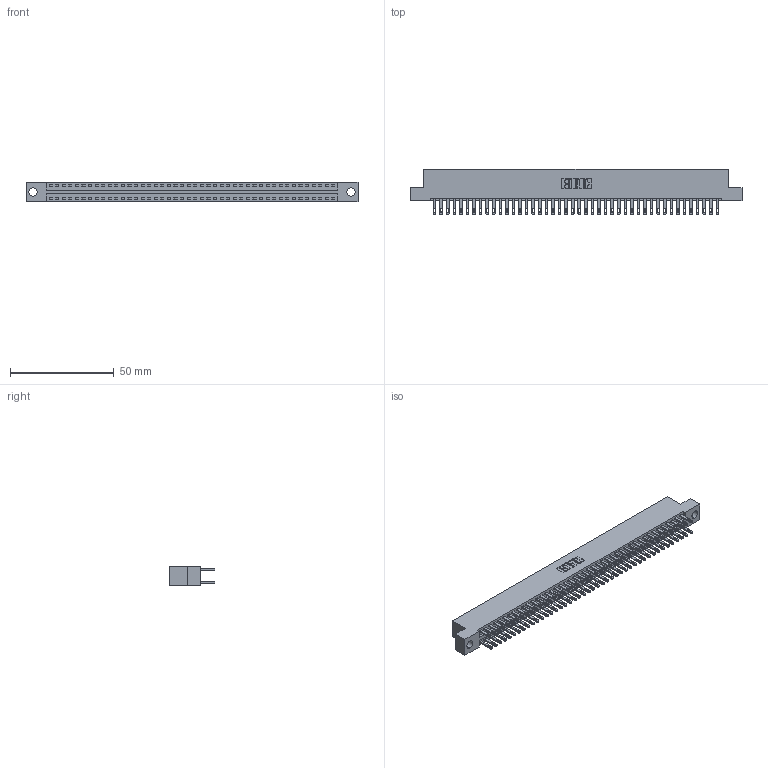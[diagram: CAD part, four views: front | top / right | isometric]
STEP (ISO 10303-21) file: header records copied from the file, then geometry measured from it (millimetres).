
FILE_DESCRIPTION (( 'STEP AP203' ), '1' );
FILE_NAME ('346-088-500-204.STEP', '2022-05-25T23:59:57', ( '' ), ( '' ), 'SwSTEP 2.0', 'SolidWorks 2020', '' );
FILE_SCHEMA (( 'CONFIG_CONTROL_DESIGN' ));
Length unit declared in the file: inch
Products named in the file (3): 346 Part_Flush Mounting Lugs - 0.156 Dia-TH; 345-292-001_345-293-100; 346-088-500-204
Assembly tree (89 placements, depth 2):
  346-088-500-204
    346 Part_Flush Mounting Lugs - 0.156 Dia-TH
    345-292-001_345-293-100  x88
Bounding box: 160.27 x 21.84 x 9.4 mm (x, y, z)
Volume: 15807.2 mm3; surface area: 22528.4 mm2
Topology: 89 solids, 89 shells, 4360 faces, 13301 edges, 8866 vertices
Faces by surface type: plane 2642, cylinder 1718
Entity records: 28795 total; most frequent: CARTESIAN_POINT 4746, ORIENTED_EDGE 4678, DIRECTION 4235, EDGE_CURVE 2339, VECTOR 2027, LINE 2027, VERTEX_POINT 1558, AXIS2_PLACEMENT_3D 1104
